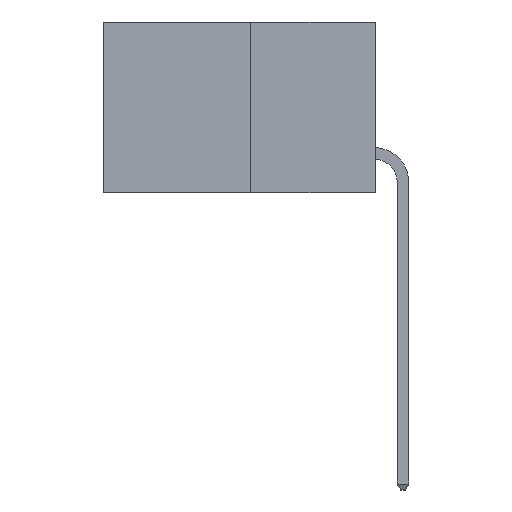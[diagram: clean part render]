
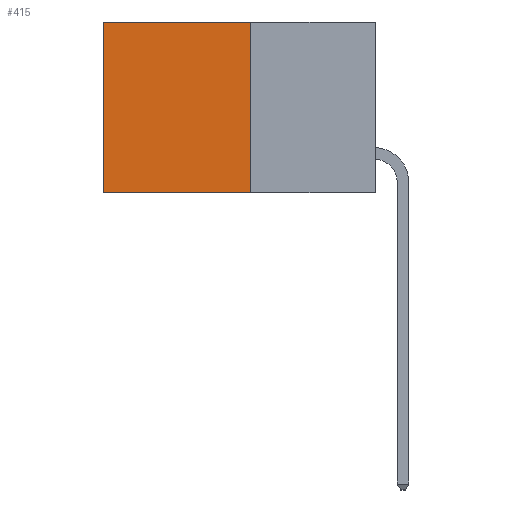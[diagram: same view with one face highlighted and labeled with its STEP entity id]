
A CAD part, left-side view. The second image highlights one B-rep face of the part: STEP entity #415.
In plain terms, the highlighted planar face has unit normal (-1, 0, 0).
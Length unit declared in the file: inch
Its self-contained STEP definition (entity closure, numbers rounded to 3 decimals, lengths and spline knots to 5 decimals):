
#143 = VECTOR ( 'NONE', #6884, 39.37008 ) ;
#209 = EDGE_LOOP ( 'NONE', ( #2162, #4674, #6730, #5596 ) ) ;
#304 = PLANE ( 'NONE',  #3809 ) ;
#415 = ADVANCED_FACE ( 'NONE', ( #4505 ), #304, .F. ) ;
#1197 = DIRECTION ( 'NONE',  ( 0., 0., -1. ) ) ;
#1613 = VERTEX_POINT ( 'NONE', #3278 ) ;
#2016 = VERTEX_POINT ( 'NONE', #4481 ) ;
#2162 = ORIENTED_EDGE ( 'NONE', *, *, #5422, .T. ) ;
#2179 = EDGE_CURVE ( 'NONE', #2016, #5146, #8938, .T. ) ;
#2410 = DIRECTION ( 'NONE',  ( 1., 0., 0. ) ) ;
#2417 = LINE ( 'NONE', #7227, #143 ) ;
#2918 = DIRECTION ( 'NONE',  ( 0., 0., -1. ) ) ;
#3267 = CARTESIAN_POINT ( 'NONE',  ( 0.277, 0.27, 0. ) ) ;
#3278 = CARTESIAN_POINT ( 'NONE',  ( 0.277, 0.27, -0.37 ) ) ;
#3413 = CARTESIAN_POINT ( 'NONE',  ( 0.277, 0.27, -0.37 ) ) ;
#3415 = VECTOR ( 'NONE', #5147, 39.37008 ) ;
#3809 = AXIS2_PLACEMENT_3D ( 'NONE', #3413, #2410, #1197 ) ;
#4481 = CARTESIAN_POINT ( 'NONE',  ( 0.277, 0.27, 0. ) ) ;
#4505 = FACE_OUTER_BOUND ( 'NONE', #209, .T. ) ;
#4674 = ORIENTED_EDGE ( 'NONE', *, *, #5711, .F. ) ;
#4985 = DIRECTION ( 'NONE',  ( 0., 1., 0. ) ) ;
#5146 = VERTEX_POINT ( 'NONE', #5854 ) ;
#5147 = DIRECTION ( 'NONE',  ( 0., 1., 0. ) ) ;
#5422 = EDGE_CURVE ( 'NONE', #5146, #7924, #2417, .T. ) ;
#5596 = ORIENTED_EDGE ( 'NONE', *, *, #2179, .T. ) ;
#5711 = EDGE_CURVE ( 'NONE', #1613, #7924, #7529, .T. ) ;
#5763 = VECTOR ( 'NONE', #4985, 39.37008 ) ;
#5854 = CARTESIAN_POINT ( 'NONE',  ( 0.277, 0.59, 0. ) ) ;
#6730 = ORIENTED_EDGE ( 'NONE', *, *, #9193, .F. ) ;
#6884 = DIRECTION ( 'NONE',  ( 0., 0., -1. ) ) ;
#6958 = LINE ( 'NONE', #7212, #8671 ) ;
#7212 = CARTESIAN_POINT ( 'NONE',  ( 0.277, 0.27, -0.37 ) ) ;
#7227 = CARTESIAN_POINT ( 'NONE',  ( 0.277, 0.59, -0.37 ) ) ;
#7512 = CARTESIAN_POINT ( 'NONE',  ( 0.277, 0.27, -0.37 ) ) ;
#7529 = LINE ( 'NONE', #7512, #5763 ) ;
#7924 = VERTEX_POINT ( 'NONE', #9246 ) ;
#8671 = VECTOR ( 'NONE', #2918, 39.37008 ) ;
#8938 = LINE ( 'NONE', #3267, #3415 ) ;
#9193 = EDGE_CURVE ( 'NONE', #2016, #1613, #6958, .T. ) ;
#9246 = CARTESIAN_POINT ( 'NONE',  ( 0.277, 0.59, -0.37 ) ) ;
